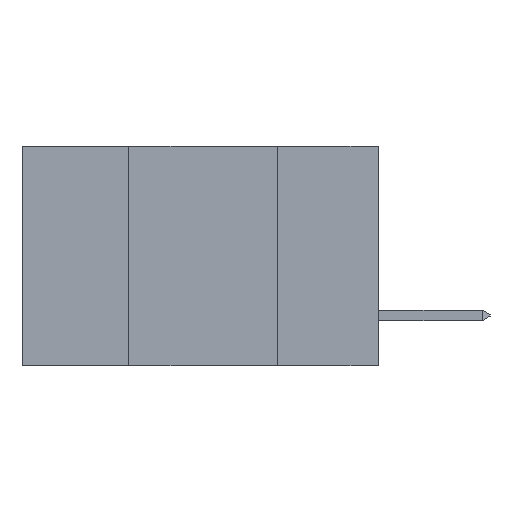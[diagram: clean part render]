
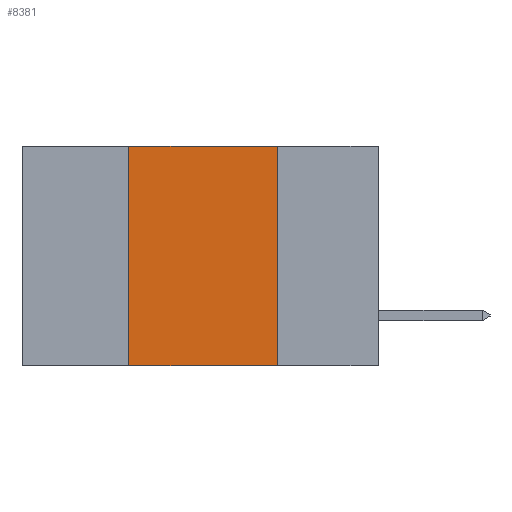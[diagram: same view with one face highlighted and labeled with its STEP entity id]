
A CAD part, left-side view. The second image highlights one B-rep face of the part: STEP entity #8381.
In plain terms, the highlighted planar face has unit normal (-1, 0, 0).
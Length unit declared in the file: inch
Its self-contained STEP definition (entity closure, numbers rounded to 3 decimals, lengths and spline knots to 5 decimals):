
#1130 = LINE ( 'NONE', #3319, #14546 ) ;
#1275 = VERTEX_POINT ( 'NONE', #4124 ) ;
#2412 = ORIENTED_EDGE ( 'NONE', *, *, #8800, .F. ) ;
#2630 = EDGE_CURVE ( 'NONE', #7758, #14657, #8946, .T. ) ;
#3146 = DIRECTION ( 'NONE',  ( 0., 0., 1. ) ) ;
#3183 = CARTESIAN_POINT ( 'NONE',  ( 0., 0.42, -0.37 ) ) ;
#3319 = CARTESIAN_POINT ( 'NONE',  ( 0., 0.6, -0.37 ) ) ;
#3808 = ORIENTED_EDGE ( 'NONE', *, *, #7047, .F. ) ;
#4124 = CARTESIAN_POINT ( 'NONE',  ( 0., 0.42, 0. ) ) ;
#4780 = CARTESIAN_POINT ( 'NONE',  ( 0., 0.17, 0. ) ) ;
#4958 = FACE_OUTER_BOUND ( 'NONE', #7651, .T. ) ;
#5008 = VECTOR ( 'NONE', #12605, 39.37008 ) ;
#5388 = VECTOR ( 'NONE', #3146, 39.37008 ) ;
#7047 = EDGE_CURVE ( 'NONE', #1275, #7758, #15264, .T. ) ;
#7168 = AXIS2_PLACEMENT_3D ( 'NONE', #12534, #12286, #12215 ) ;
#7566 = ORIENTED_EDGE ( 'NONE', *, *, #11344, .T. ) ;
#7651 = EDGE_LOOP ( 'NONE', ( #9561, #3808, #2412, #7566 ) ) ;
#7758 = VERTEX_POINT ( 'NONE', #4780 ) ;
#8381 = ADVANCED_FACE ( 'NONE', ( #4958 ), #12890, .F. ) ;
#8800 = EDGE_CURVE ( 'NONE', #15968, #1275, #15575, .T. ) ;
#8946 = LINE ( 'NONE', #13916, #15298 ) ;
#9561 = ORIENTED_EDGE ( 'NONE', *, *, #2630, .F. ) ;
#10440 = CARTESIAN_POINT ( 'NONE',  ( 0., 0.42, -0.37 ) ) ;
#11344 = EDGE_CURVE ( 'NONE', #15968, #14657, #1130, .T. ) ;
#12152 = CARTESIAN_POINT ( 'NONE',  ( 0., 0.17, -0.37 ) ) ;
#12215 = DIRECTION ( 'NONE',  ( 0., 0., -1. ) ) ;
#12286 = DIRECTION ( 'NONE',  ( 1., 0., 0. ) ) ;
#12534 = CARTESIAN_POINT ( 'NONE',  ( 0., 0.6, 0. ) ) ;
#12605 = DIRECTION ( 'NONE',  ( 0., -1., 0. ) ) ;
#12684 = CARTESIAN_POINT ( 'NONE',  ( 0., 0.6, 0. ) ) ;
#12890 = PLANE ( 'NONE',  #7168 ) ;
#13898 = DIRECTION ( 'NONE',  ( 0., 0., -1. ) ) ;
#13916 = CARTESIAN_POINT ( 'NONE',  ( 0., 0.17, -0.37 ) ) ;
#14546 = VECTOR ( 'NONE', #14963, 39.37008 ) ;
#14657 = VERTEX_POINT ( 'NONE', #12152 ) ;
#14963 = DIRECTION ( 'NONE',  ( 0., -1., 0. ) ) ;
#15264 = LINE ( 'NONE', #12684, #5008 ) ;
#15298 = VECTOR ( 'NONE', #13898, 39.37008 ) ;
#15575 = LINE ( 'NONE', #3183, #5388 ) ;
#15968 = VERTEX_POINT ( 'NONE', #10440 ) ;
